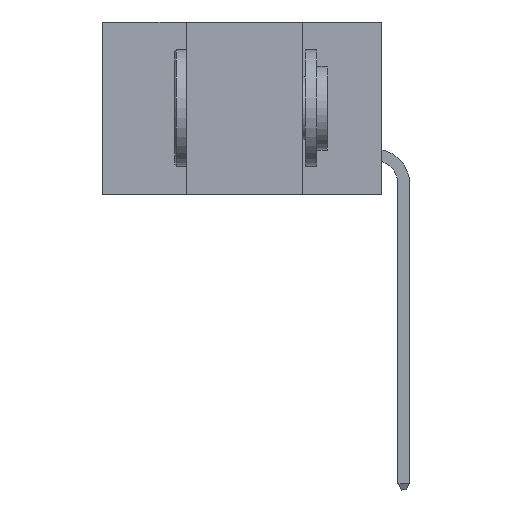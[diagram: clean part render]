
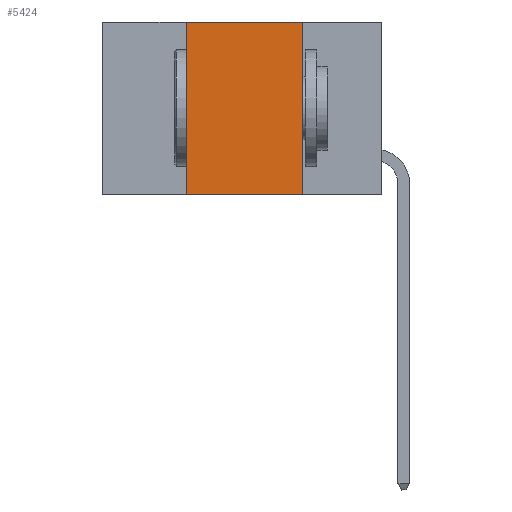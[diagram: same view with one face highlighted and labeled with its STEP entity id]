
A CAD part, left-side view. The second image highlights one B-rep face of the part: STEP entity #5424.
In plain terms, the highlighted planar face has unit normal (-1, 0, 0).
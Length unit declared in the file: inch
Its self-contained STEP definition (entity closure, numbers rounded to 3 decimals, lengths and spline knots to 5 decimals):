
#2471 = EDGE_CURVE ( 'NONE', #17754, #17570, #13540, .T. ) ;
#3011 = EDGE_CURVE ( 'NONE', #10048, #17754, #12102, .T. ) ;
#3263 = LINE ( 'NONE', #15817, #10346 ) ;
#3439 = ORIENTED_EDGE ( 'NONE', *, *, #8983, .F. ) ;
#4951 = EDGE_LOOP ( 'NONE', ( #12678, #6116, #3439, #10348 ) ) ;
#5424 = ADVANCED_FACE ( 'NONE', ( #17073 ), #16867, .F. ) ;
#6116 = ORIENTED_EDGE ( 'NONE', *, *, #3011, .F. ) ;
#6257 = DIRECTION ( 'NONE',  ( 0., 0., -1. ) ) ;
#7133 = DIRECTION ( 'NONE',  ( 0., -1., 0. ) ) ;
#7480 = CARTESIAN_POINT ( 'NONE',  ( 0., 0.42, 0. ) ) ;
#8102 = CARTESIAN_POINT ( 'NONE',  ( 0., 0.17, 0. ) ) ;
#8410 = VECTOR ( 'NONE', #19022, 39.37008 ) ;
#8983 = EDGE_CURVE ( 'NONE', #10592, #10048, #15295, .T. ) ;
#9528 = CARTESIAN_POINT ( 'NONE',  ( 0., 0.17, 0. ) ) ;
#9710 = DIRECTION ( 'NONE',  ( 0., -1., 0. ) ) ;
#9714 = VECTOR ( 'NONE', #9710, 39.37008 ) ;
#10048 = VERTEX_POINT ( 'NONE', #17776 ) ;
#10346 = VECTOR ( 'NONE', #7133, 39.37008 ) ;
#10348 = ORIENTED_EDGE ( 'NONE', *, *, #11841, .T. ) ;
#10592 = VERTEX_POINT ( 'NONE', #12377 ) ;
#11841 = EDGE_CURVE ( 'NONE', #10592, #17570, #3263, .T. ) ;
#12102 = LINE ( 'NONE', #16828, #9714 ) ;
#12377 = CARTESIAN_POINT ( 'NONE',  ( 0., 0.42, -0.37 ) ) ;
#12678 = ORIENTED_EDGE ( 'NONE', *, *, #2471, .F. ) ;
#13540 = LINE ( 'NONE', #8102, #13869 ) ;
#13869 = VECTOR ( 'NONE', #6257, 39.37008 ) ;
#15295 = LINE ( 'NONE', #7480, #8410 ) ;
#15817 = CARTESIAN_POINT ( 'NONE',  ( 0., 0.6, -0.37 ) ) ;
#16828 = CARTESIAN_POINT ( 'NONE',  ( 0., 0.6, 0. ) ) ;
#16867 = PLANE ( 'NONE',  #19498 ) ;
#17073 = FACE_OUTER_BOUND ( 'NONE', #4951, .T. ) ;
#17308 = CARTESIAN_POINT ( 'NONE',  ( 0., 0.6, 0. ) ) ;
#17536 = DIRECTION ( 'NONE',  ( 0., 0., -1. ) ) ;
#17570 = VERTEX_POINT ( 'NONE', #18104 ) ;
#17754 = VERTEX_POINT ( 'NONE', #9528 ) ;
#17776 = CARTESIAN_POINT ( 'NONE',  ( 0., 0.42, 0. ) ) ;
#18104 = CARTESIAN_POINT ( 'NONE',  ( 0., 0.17, -0.37 ) ) ;
#19022 = DIRECTION ( 'NONE',  ( 0., 0., 1. ) ) ;
#19498 = AXIS2_PLACEMENT_3D ( 'NONE', #17308, #20690, #17536 ) ;
#20690 = DIRECTION ( 'NONE',  ( 1., 0., 0. ) ) ;
